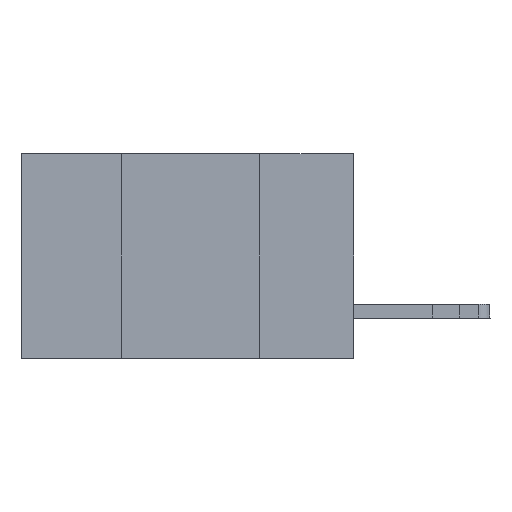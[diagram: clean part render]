
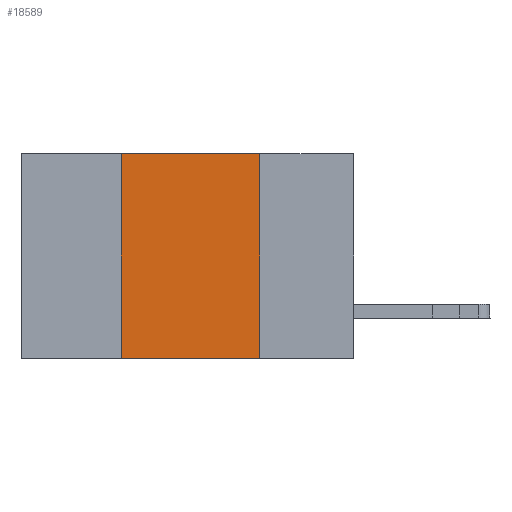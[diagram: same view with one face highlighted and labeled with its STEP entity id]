
A CAD part, left-side view. The second image highlights one B-rep face of the part: STEP entity #18589.
In plain terms, the highlighted planar face has unit normal (-1, 0, 0).
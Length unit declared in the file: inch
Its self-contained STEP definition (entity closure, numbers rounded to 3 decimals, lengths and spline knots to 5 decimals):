
#873 = CARTESIAN_POINT ( 'NONE',  ( 0., 0.42, -0.37 ) ) ;
#997 = DIRECTION ( 'NONE',  ( 0., -1., 0. ) ) ;
#1397 = ORIENTED_EDGE ( 'NONE', *, *, #26263, .F. ) ;
#1712 = DIRECTION ( 'NONE',  ( 0., 0., -1. ) ) ;
#1931 = DIRECTION ( 'NONE',  ( 0., 0., 1. ) ) ;
#2974 = DIRECTION ( 'NONE',  ( 0., 0., -1. ) ) ;
#3064 = CARTESIAN_POINT ( 'NONE',  ( 0., 0.6, 0. ) ) ;
#3623 = CARTESIAN_POINT ( 'NONE',  ( 0., 0.42, 0. ) ) ;
#4258 = VECTOR ( 'NONE', #1712, 39.37008 ) ;
#8279 = ORIENTED_EDGE ( 'NONE', *, *, #21087, .F. ) ;
#8387 = VECTOR ( 'NONE', #25114, 39.37008 ) ;
#9072 = ORIENTED_EDGE ( 'NONE', *, *, #17206, .T. ) ;
#9912 = VERTEX_POINT ( 'NONE', #13153 ) ;
#10565 = VECTOR ( 'NONE', #997, 39.37008 ) ;
#10709 = VERTEX_POINT ( 'NONE', #12335 ) ;
#10876 = FACE_OUTER_BOUND ( 'NONE', #19511, .T. ) ;
#11215 = ORIENTED_EDGE ( 'NONE', *, *, #11551, .F. ) ;
#11551 = EDGE_CURVE ( 'NONE', #10709, #9912, #14099, .T. ) ;
#11742 = LINE ( 'NONE', #3623, #17873 ) ;
#12335 = CARTESIAN_POINT ( 'NONE',  ( 0., 0.42, 0. ) ) ;
#13153 = CARTESIAN_POINT ( 'NONE',  ( 0., 0.17, 0. ) ) ;
#13313 = CARTESIAN_POINT ( 'NONE',  ( 0., 0.6, 0. ) ) ;
#13401 = PLANE ( 'NONE',  #26641 ) ;
#14099 = LINE ( 'NONE', #13313, #10565 ) ;
#15182 = LINE ( 'NONE', #24313, #4258 ) ;
#15307 = VERTEX_POINT ( 'NONE', #873 ) ;
#17206 = EDGE_CURVE ( 'NONE', #15307, #21727, #19373, .T. ) ;
#17873 = VECTOR ( 'NONE', #1931, 39.37008 ) ;
#18084 = CARTESIAN_POINT ( 'NONE',  ( 0., 0.17, -0.37 ) ) ;
#18589 = ADVANCED_FACE ( 'NONE', ( #10876 ), #13401, .F. ) ;
#19373 = LINE ( 'NONE', #21046, #8387 ) ;
#19511 = EDGE_LOOP ( 'NONE', ( #1397, #11215, #8279, #9072 ) ) ;
#21046 = CARTESIAN_POINT ( 'NONE',  ( 0., 0.6, -0.37 ) ) ;
#21087 = EDGE_CURVE ( 'NONE', #15307, #10709, #11742, .T. ) ;
#21727 = VERTEX_POINT ( 'NONE', #18084 ) ;
#24313 = CARTESIAN_POINT ( 'NONE',  ( 0., 0.17, 0. ) ) ;
#25114 = DIRECTION ( 'NONE',  ( 0., -1., 0. ) ) ;
#25846 = DIRECTION ( 'NONE',  ( 1., 0., 0. ) ) ;
#26263 = EDGE_CURVE ( 'NONE', #9912, #21727, #15182, .T. ) ;
#26641 = AXIS2_PLACEMENT_3D ( 'NONE', #3064, #25846, #2974 ) ;
